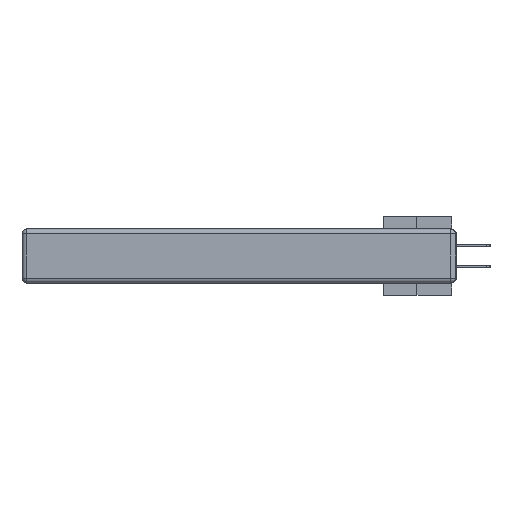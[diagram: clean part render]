
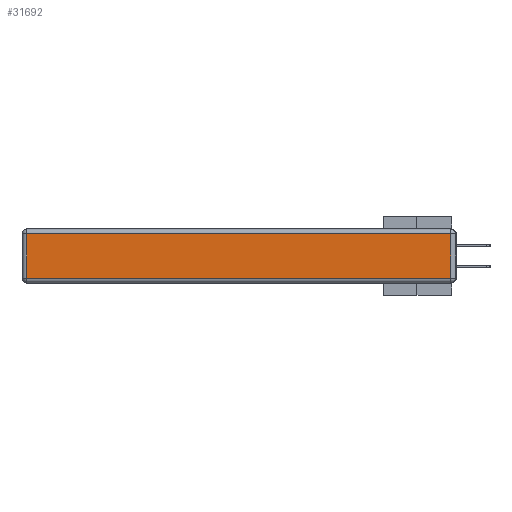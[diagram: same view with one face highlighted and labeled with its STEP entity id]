
A CAD part, left-side view. The second image highlights one B-rep face of the part: STEP entity #31692.
In plain terms, the highlighted planar face has unit normal (-1, 0, 0).
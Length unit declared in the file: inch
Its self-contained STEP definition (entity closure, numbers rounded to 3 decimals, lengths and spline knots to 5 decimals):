
#22 = CARTESIAN_POINT ( 'NONE',  ( 0., 2.75, -0.03 ) ) ;
#1087 = EDGE_CURVE ( 'NONE', #8338, #9440, #20453, .T. ) ;
#1531 = EDGE_CURVE ( 'NONE', #13367, #8338, #39332, .T. ) ;
#2632 = DIRECTION ( 'NONE',  ( 0., 1., 0. ) ) ;
#2699 = CARTESIAN_POINT ( 'NONE',  ( 0., 2.72, -0.313 ) ) ;
#3991 = VECTOR ( 'NONE', #2632, 39.37008 ) ;
#4155 = VECTOR ( 'NONE', #39987, 39.37008 ) ;
#5289 = EDGE_CURVE ( 'NONE', #29296, #13367, #36608, .T. ) ;
#5796 = FACE_OUTER_BOUND ( 'NONE', #15476, .T. ) ;
#7287 = DIRECTION ( 'NONE',  ( 0., 0., 1. ) ) ;
#8338 = VERTEX_POINT ( 'NONE', #2699 ) ;
#9440 = VERTEX_POINT ( 'NONE', #16633 ) ;
#11381 = PLANE ( 'NONE',  #42184 ) ;
#11517 = DIRECTION ( 'NONE',  ( 0., 0., 1. ) ) ;
#13367 = VERTEX_POINT ( 'NONE', #26758 ) ;
#13824 = EDGE_CURVE ( 'NONE', #9440, #29296, #37275, .T. ) ;
#15476 = EDGE_LOOP ( 'NONE', ( #39606, #33553, #34259, #36149 ) ) ;
#16633 = CARTESIAN_POINT ( 'NONE',  ( 0., 0.03, -0.313 ) ) ;
#17844 = VECTOR ( 'NONE', #23107, 39.37008 ) ;
#20453 = LINE ( 'NONE', #26978, #4155 ) ;
#21449 = VECTOR ( 'NONE', #7287, 39.37008 ) ;
#23107 = DIRECTION ( 'NONE',  ( 0., 0., -1. ) ) ;
#26758 = CARTESIAN_POINT ( 'NONE',  ( 0., 2.72, -0.03 ) ) ;
#26978 = CARTESIAN_POINT ( 'NONE',  ( 0., 0., -0.313 ) ) ;
#29296 = VERTEX_POINT ( 'NONE', #30391 ) ;
#29850 = CARTESIAN_POINT ( 'NONE',  ( 0., 0.03, -0.343 ) ) ;
#30391 = CARTESIAN_POINT ( 'NONE',  ( 0., 0.03, -0.03 ) ) ;
#31692 = ADVANCED_FACE ( 'NONE', ( #5796 ), #11381, .T. ) ;
#32517 = CARTESIAN_POINT ( 'NONE',  ( 0., 2.72, -0.343 ) ) ;
#33553 = ORIENTED_EDGE ( 'NONE', *, *, #13824, .T. ) ;
#34235 = DIRECTION ( 'NONE',  ( -1., 0., 0. ) ) ;
#34259 = ORIENTED_EDGE ( 'NONE', *, *, #5289, .T. ) ;
#36149 = ORIENTED_EDGE ( 'NONE', *, *, #1531, .T. ) ;
#36608 = LINE ( 'NONE', #22, #3991 ) ;
#37275 = LINE ( 'NONE', #29850, #21449 ) ;
#39332 = LINE ( 'NONE', #32517, #17844 ) ;
#39606 = ORIENTED_EDGE ( 'NONE', *, *, #1087, .T. ) ;
#39987 = DIRECTION ( 'NONE',  ( 0., -1., 0. ) ) ;
#41283 = CARTESIAN_POINT ( 'NONE',  ( 0., 0., -0.343 ) ) ;
#42184 = AXIS2_PLACEMENT_3D ( 'NONE', #41283, #34235, #11517 ) ;
